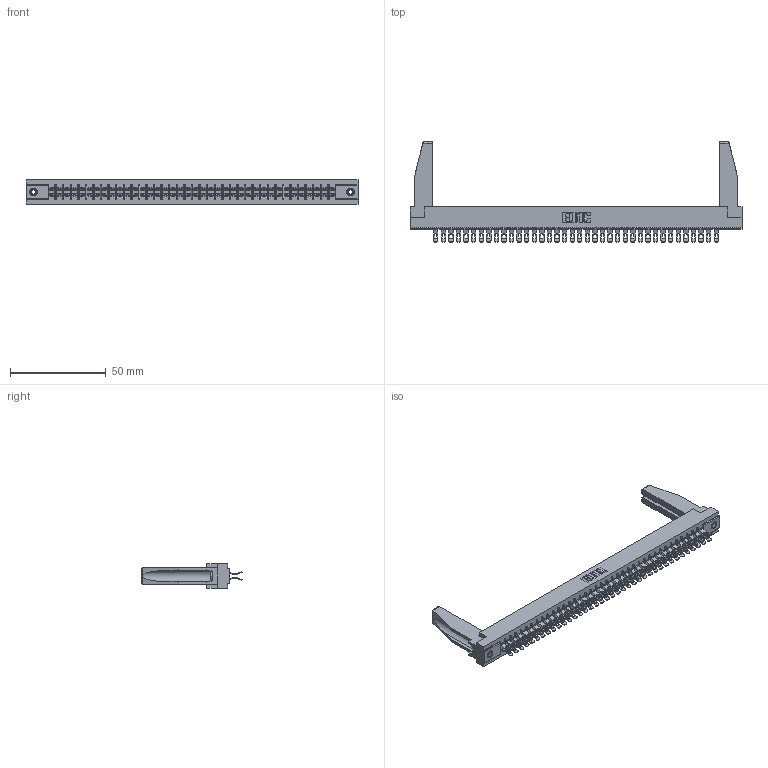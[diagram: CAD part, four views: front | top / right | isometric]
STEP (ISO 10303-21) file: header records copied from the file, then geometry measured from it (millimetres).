
FILE_DESCRIPTION (( 'STEP AP203' ), '1' );
FILE_NAME ('315-076-555-278.STEP', '2019-09-10T22:35:09', ( '' ), ( '' ), 'SwSTEP 2.0', 'SolidWorks 2016', '' );
FILE_SCHEMA (( 'CONFIG_CONTROL_DESIGN' ));
Length unit declared in the file: inch
Products named in the file (5): 307-220-078; 315-076-555-278; 305-290-001_555; 345-250-001_345-250-001-102; 305 Part_.156 Dia
Assembly tree (81 placements, depth 2):
  315-076-555-278
    305 Part_.156 Dia
    305-290-001_555  x76
    345-250-001_345-250-001-102  x2
    307-220-078  x2
Bounding box: 173.58 x 52.45 x 12.7 mm (x, y, z)
Volume: 22304.8 mm3; surface area: 28457.2 mm2
Topology: 81 solids, 81 shells, 5262 faces, 15656 edges, 10224 vertices
Faces by surface type: plane 2584, cylinder 2510, sphere 152, cone 12, torus 4
Entity records: 44694 total; most frequent: CARTESIAN_POINT 7420, ORIENTED_EDGE 7314, DIRECTION 7133, EDGE_CURVE 3657, VECTOR 2931, LINE 2931, VERTEX_POINT 2330, AXIS2_PLACEMENT_3D 2101
